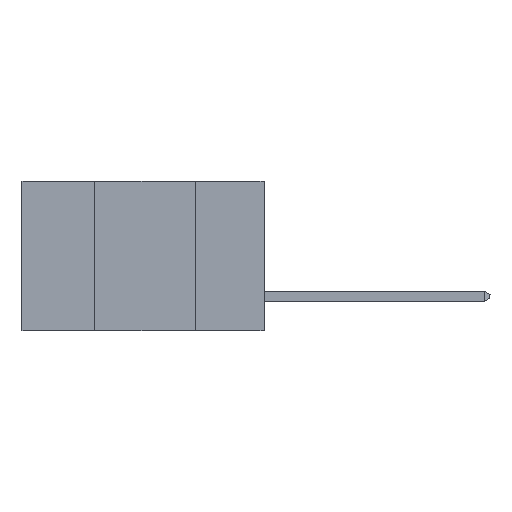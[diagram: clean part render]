
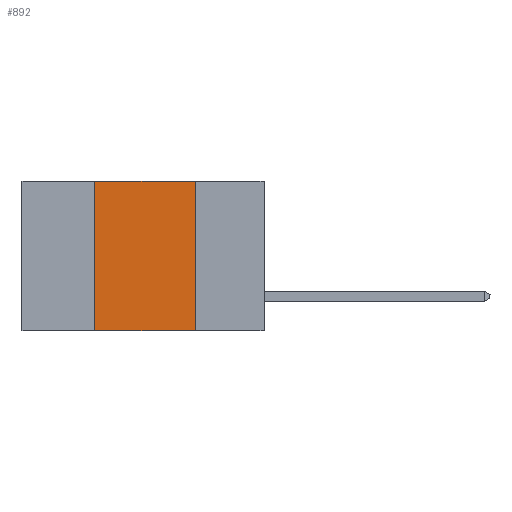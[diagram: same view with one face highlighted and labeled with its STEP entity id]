
A CAD part, left-side view. The second image highlights one B-rep face of the part: STEP entity #892.
In plain terms, the highlighted planar face has unit normal (-1, 0, 0).
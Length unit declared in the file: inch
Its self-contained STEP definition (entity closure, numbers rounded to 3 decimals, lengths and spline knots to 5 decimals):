
#90 = EDGE_CURVE ( 'NONE', #1170, #12769, #4068, .T. ) ;
#892 = ADVANCED_FACE ( 'NONE', ( #17872 ), #4520, .F. ) ;
#1086 = LINE ( 'NONE', #9617, #16932 ) ;
#1170 = VERTEX_POINT ( 'NONE', #4428 ) ;
#1605 = LINE ( 'NONE', #2025, #2723 ) ;
#2025 = CARTESIAN_POINT ( 'NONE',  ( 0., 0.6, -0.37 ) ) ;
#2129 = ORIENTED_EDGE ( 'NONE', *, *, #90, .F. ) ;
#2199 = VERTEX_POINT ( 'NONE', #17384 ) ;
#2723 = VECTOR ( 'NONE', #13524, 39.37008 ) ;
#2801 = EDGE_LOOP ( 'NONE', ( #10881, #2129, #15230, #17611 ) ) ;
#3514 = CARTESIAN_POINT ( 'NONE',  ( 0., 0.6, 0. ) ) ;
#3849 = DIRECTION ( 'NONE',  ( 0., 0., 1. ) ) ;
#4040 = CARTESIAN_POINT ( 'NONE',  ( 0., 0.17, 0. ) ) ;
#4068 = LINE ( 'NONE', #3514, #8796 ) ;
#4384 = CARTESIAN_POINT ( 'NONE',  ( 0., 0.17, 0. ) ) ;
#4428 = CARTESIAN_POINT ( 'NONE',  ( 0., 0.42, 0. ) ) ;
#4520 = PLANE ( 'NONE',  #5495 ) ;
#5353 = LINE ( 'NONE', #4384, #5591 ) ;
#5495 = AXIS2_PLACEMENT_3D ( 'NONE', #8935, #5971, #15879 ) ;
#5591 = VECTOR ( 'NONE', #7188, 39.37008 ) ;
#5717 = VERTEX_POINT ( 'NONE', #9807 ) ;
#5971 = DIRECTION ( 'NONE',  ( 1., 0., 0. ) ) ;
#7188 = DIRECTION ( 'NONE',  ( 0., 0., -1. ) ) ;
#7288 = EDGE_CURVE ( 'NONE', #5717, #2199, #1605, .T. ) ;
#8796 = VECTOR ( 'NONE', #13703, 39.37008 ) ;
#8935 = CARTESIAN_POINT ( 'NONE',  ( 0., 0.6, 0. ) ) ;
#9617 = CARTESIAN_POINT ( 'NONE',  ( 0., 0.42, 0. ) ) ;
#9807 = CARTESIAN_POINT ( 'NONE',  ( 0., 0.42, -0.37 ) ) ;
#10881 = ORIENTED_EDGE ( 'NONE', *, *, #12167, .F. ) ;
#12167 = EDGE_CURVE ( 'NONE', #12769, #2199, #5353, .T. ) ;
#12769 = VERTEX_POINT ( 'NONE', #4040 ) ;
#12785 = EDGE_CURVE ( 'NONE', #5717, #1170, #1086, .T. ) ;
#13524 = DIRECTION ( 'NONE',  ( 0., -1., 0. ) ) ;
#13703 = DIRECTION ( 'NONE',  ( 0., -1., 0. ) ) ;
#15230 = ORIENTED_EDGE ( 'NONE', *, *, #12785, .F. ) ;
#15879 = DIRECTION ( 'NONE',  ( 0., 0., -1. ) ) ;
#16932 = VECTOR ( 'NONE', #3849, 39.37008 ) ;
#17384 = CARTESIAN_POINT ( 'NONE',  ( 0., 0.17, -0.37 ) ) ;
#17611 = ORIENTED_EDGE ( 'NONE', *, *, #7288, .T. ) ;
#17872 = FACE_OUTER_BOUND ( 'NONE', #2801, .T. ) ;
